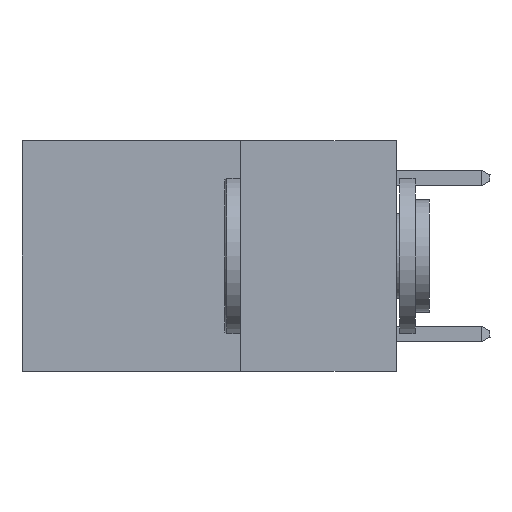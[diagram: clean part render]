
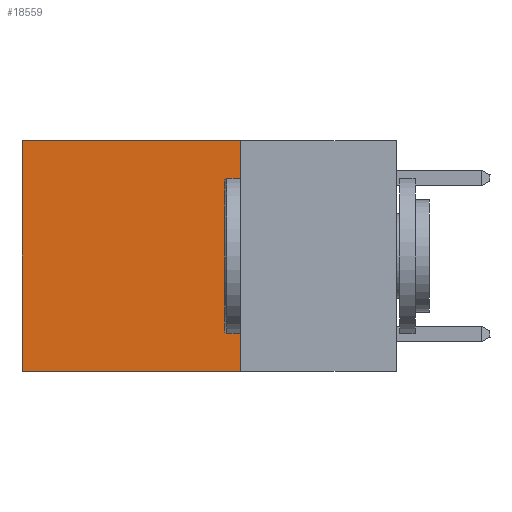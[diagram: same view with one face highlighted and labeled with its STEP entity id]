
A CAD part, left-side view. The second image highlights one B-rep face of the part: STEP entity #18559.
In plain terms, the highlighted planar face has unit normal (-1, 0, 0).
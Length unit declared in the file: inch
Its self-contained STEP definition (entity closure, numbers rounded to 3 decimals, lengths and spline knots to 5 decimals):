
#839 = AXIS2_PLACEMENT_3D ( 'NONE', #19047, #9726, #15266 ) ;
#1451 = ORIENTED_EDGE ( 'NONE', *, *, #22590, .T. ) ;
#1474 = ORIENTED_EDGE ( 'NONE', *, *, #2005, .T. ) ;
#1948 = VERTEX_POINT ( 'NONE', #21454 ) ;
#2005 = EDGE_CURVE ( 'NONE', #13203, #23318, #12049, .T. ) ;
#3590 = EDGE_CURVE ( 'NONE', #1948, #9162, #15610, .T. ) ;
#5109 = LINE ( 'NONE', #22020, #6444 ) ;
#6095 = DIRECTION ( 'NONE',  ( 0., 1., 0. ) ) ;
#6245 = VECTOR ( 'NONE', #6095, 39.37008 ) ;
#6444 = VECTOR ( 'NONE', #20380, 39.37008 ) ;
#7857 = LINE ( 'NONE', #15379, #6245 ) ;
#7867 = FACE_OUTER_BOUND ( 'NONE', #15511, .T. ) ;
#9162 = VERTEX_POINT ( 'NONE', #18211 ) ;
#9361 = PLANE ( 'NONE',  #839 ) ;
#9726 = DIRECTION ( 'NONE',  ( 1., 0., 0. ) ) ;
#9941 = CARTESIAN_POINT ( 'NONE',  ( 0.2625, 0.25, 0. ) ) ;
#11970 = VECTOR ( 'NONE', #23308, 39.37008 ) ;
#12049 = LINE ( 'NONE', #17738, #11970 ) ;
#12840 = ORIENTED_EDGE ( 'NONE', *, *, #14307, .F. ) ;
#12961 = CARTESIAN_POINT ( 'NONE',  ( 0.2625, 0.6, 0. ) ) ;
#13203 = VERTEX_POINT ( 'NONE', #12961 ) ;
#13634 = DIRECTION ( 'NONE',  ( 0., 0., -1. ) ) ;
#14307 = EDGE_CURVE ( 'NONE', #9162, #23318, #7857, .T. ) ;
#15266 = DIRECTION ( 'NONE',  ( 0., 0., -1. ) ) ;
#15379 = CARTESIAN_POINT ( 'NONE',  ( 0.2625, 0.25, -0.37 ) ) ;
#15511 = EDGE_LOOP ( 'NONE', ( #1474, #12840, #21472, #1451 ) ) ;
#15610 = LINE ( 'NONE', #9941, #22662 ) ;
#17738 = CARTESIAN_POINT ( 'NONE',  ( 0.2625, 0.6, 0. ) ) ;
#18211 = CARTESIAN_POINT ( 'NONE',  ( 0.2625, 0.25, -0.37 ) ) ;
#18559 = ADVANCED_FACE ( 'NONE', ( #7867 ), #9361, .F. ) ;
#19047 = CARTESIAN_POINT ( 'NONE',  ( 0.2625, 0.25, 0. ) ) ;
#20380 = DIRECTION ( 'NONE',  ( 0., 1., 0. ) ) ;
#21454 = CARTESIAN_POINT ( 'NONE',  ( 0.2625, 0.25, 0. ) ) ;
#21472 = ORIENTED_EDGE ( 'NONE', *, *, #3590, .F. ) ;
#22020 = CARTESIAN_POINT ( 'NONE',  ( 0.2625, 0.25, 0. ) ) ;
#22590 = EDGE_CURVE ( 'NONE', #1948, #13203, #5109, .T. ) ;
#22662 = VECTOR ( 'NONE', #13634, 39.37008 ) ;
#23308 = DIRECTION ( 'NONE',  ( 0., 0., -1. ) ) ;
#23318 = VERTEX_POINT ( 'NONE', #24026 ) ;
#24026 = CARTESIAN_POINT ( 'NONE',  ( 0.2625, 0.6, -0.37 ) ) ;
